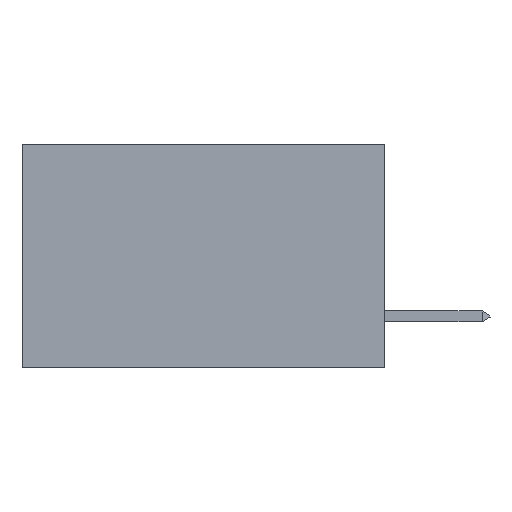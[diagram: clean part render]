
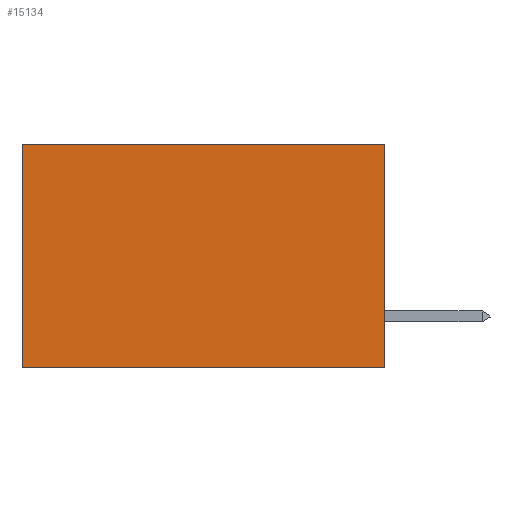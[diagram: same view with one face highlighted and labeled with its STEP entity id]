
A CAD part, left-side view. The second image highlights one B-rep face of the part: STEP entity #15134.
In plain terms, the highlighted planar face has unit normal (-1, 0, 0).
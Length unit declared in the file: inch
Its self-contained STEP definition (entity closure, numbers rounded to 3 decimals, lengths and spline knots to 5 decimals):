
#1983 = EDGE_CURVE ( 'NONE', #21049, #13522, #18401, .T. ) ;
#2079 = DIRECTION ( 'NONE',  ( 0., 1., 0. ) ) ;
#4045 = LINE ( 'NONE', #26923, #19379 ) ;
#4324 = CARTESIAN_POINT ( 'NONE',  ( 0.2875, 0., 0. ) ) ;
#4779 = VECTOR ( 'NONE', #11575, 39.37008 ) ;
#5662 = PLANE ( 'NONE',  #18468 ) ;
#7515 = DIRECTION ( 'NONE',  ( 0., 0., -1. ) ) ;
#8108 = DIRECTION ( 'NONE',  ( 0., 0., -1. ) ) ;
#8926 = LINE ( 'NONE', #17687, #13354 ) ;
#10416 = CARTESIAN_POINT ( 'NONE',  ( 0.2875, 0.6, 0. ) ) ;
#10853 = ORIENTED_EDGE ( 'NONE', *, *, #19019, .F. ) ;
#11575 = DIRECTION ( 'NONE',  ( 0., 0., -1. ) ) ;
#11604 = EDGE_CURVE ( 'NONE', #25427, #21049, #8926, .T. ) ;
#11868 = FACE_OUTER_BOUND ( 'NONE', #13784, .T. ) ;
#12152 = CARTESIAN_POINT ( 'NONE',  ( 0.2875, 0.6, -0.37 ) ) ;
#13354 = VECTOR ( 'NONE', #2079, 39.37008 ) ;
#13522 = VERTEX_POINT ( 'NONE', #12152 ) ;
#13543 = EDGE_CURVE ( 'NONE', #24751, #13522, #4045, .T. ) ;
#13784 = EDGE_LOOP ( 'NONE', ( #14803, #28423, #10853, #25811 ) ) ;
#13860 = CARTESIAN_POINT ( 'NONE',  ( 0.2875, 0., 0. ) ) ;
#14803 = ORIENTED_EDGE ( 'NONE', *, *, #1983, .T. ) ;
#15134 = ADVANCED_FACE ( 'NONE', ( #11868 ), #5662, .F. ) ;
#16856 = DIRECTION ( 'NONE',  ( 0., 1., 0. ) ) ;
#17375 = CARTESIAN_POINT ( 'NONE',  ( 0.2875, 0., 0. ) ) ;
#17687 = CARTESIAN_POINT ( 'NONE',  ( 0.2875, 0., 0. ) ) ;
#17974 = CARTESIAN_POINT ( 'NONE',  ( 0.2875, 0., -0.37 ) ) ;
#18317 = LINE ( 'NONE', #4324, #4779 ) ;
#18401 = LINE ( 'NONE', #24487, #30058 ) ;
#18468 = AXIS2_PLACEMENT_3D ( 'NONE', #17375, #19526, #8108 ) ;
#19019 = EDGE_CURVE ( 'NONE', #25427, #24751, #18317, .T. ) ;
#19379 = VECTOR ( 'NONE', #16856, 39.37008 ) ;
#19526 = DIRECTION ( 'NONE',  ( 1., 0., 0. ) ) ;
#21049 = VERTEX_POINT ( 'NONE', #10416 ) ;
#24487 = CARTESIAN_POINT ( 'NONE',  ( 0.2875, 0.6, 0. ) ) ;
#24751 = VERTEX_POINT ( 'NONE', #17974 ) ;
#25427 = VERTEX_POINT ( 'NONE', #13860 ) ;
#25811 = ORIENTED_EDGE ( 'NONE', *, *, #11604, .T. ) ;
#26923 = CARTESIAN_POINT ( 'NONE',  ( 0.2875, 0., -0.37 ) ) ;
#28423 = ORIENTED_EDGE ( 'NONE', *, *, #13543, .F. ) ;
#30058 = VECTOR ( 'NONE', #7515, 39.37008 ) ;
